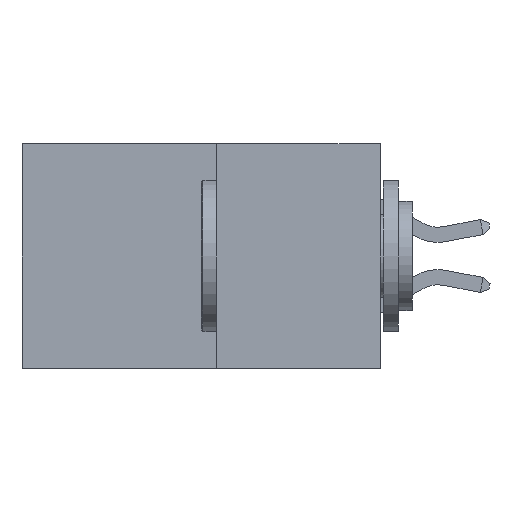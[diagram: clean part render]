
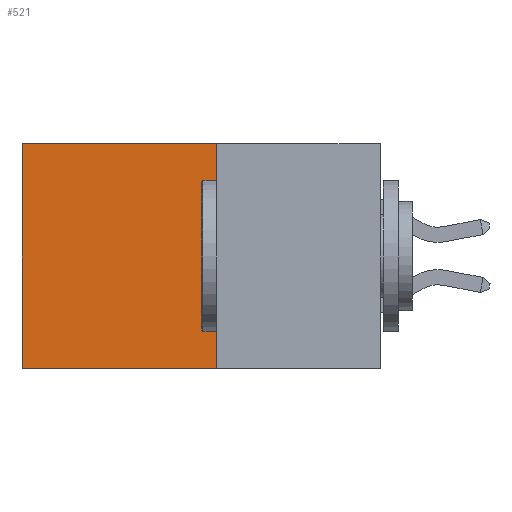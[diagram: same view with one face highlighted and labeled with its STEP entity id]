
A CAD part, left-side view. The second image highlights one B-rep face of the part: STEP entity #521.
In plain terms, the highlighted planar face has unit normal (-1, 0, 0).
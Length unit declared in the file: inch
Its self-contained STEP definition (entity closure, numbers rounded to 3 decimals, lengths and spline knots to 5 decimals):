
#521 = ADVANCED_FACE ( 'NONE', ( #11452 ), #2198, .F. ) ;
#563 = LINE ( 'NONE', #14332, #9038 ) ;
#1835 = VERTEX_POINT ( 'NONE', #4937 ) ;
#1877 = LINE ( 'NONE', #12986, #18671 ) ;
#2198 = PLANE ( 'NONE',  #16958 ) ;
#2316 = VECTOR ( 'NONE', #6111, 39.37008 ) ;
#2843 = LINE ( 'NONE', #6462, #2316 ) ;
#2913 = ORIENTED_EDGE ( 'NONE', *, *, #20749, .T. ) ;
#3268 = CARTESIAN_POINT ( 'NONE',  ( 0.277, 0.59, -0.37 ) ) ;
#3866 = ORIENTED_EDGE ( 'NONE', *, *, #10533, .T. ) ;
#4174 = EDGE_LOOP ( 'NONE', ( #3866, #16039, #15966, #2913 ) ) ;
#4552 = DIRECTION ( 'NONE',  ( 0., 1., 0. ) ) ;
#4937 = CARTESIAN_POINT ( 'NONE',  ( 0.277, 0.59, 0. ) ) ;
#6039 = DIRECTION ( 'NONE',  ( 1., 0., 0. ) ) ;
#6047 = CARTESIAN_POINT ( 'NONE',  ( 0.277, 0.27, -0.37 ) ) ;
#6111 = DIRECTION ( 'NONE',  ( 0., 0., -1. ) ) ;
#6462 = CARTESIAN_POINT ( 'NONE',  ( 0.277, 0.59, -0.37 ) ) ;
#7021 = CARTESIAN_POINT ( 'NONE',  ( 0.277, 0.27, -0.37 ) ) ;
#7268 = VECTOR ( 'NONE', #20323, 39.37008 ) ;
#9038 = VECTOR ( 'NONE', #11083, 39.37008 ) ;
#10260 = VERTEX_POINT ( 'NONE', #12584 ) ;
#10533 = EDGE_CURVE ( 'NONE', #1835, #16772, #2843, .T. ) ;
#10762 = CARTESIAN_POINT ( 'NONE',  ( 0.277, 0.27, 0. ) ) ;
#11035 = DIRECTION ( 'NONE',  ( 0., 0., -1. ) ) ;
#11083 = DIRECTION ( 'NONE',  ( 0., 1., 0. ) ) ;
#11452 = FACE_OUTER_BOUND ( 'NONE', #4174, .T. ) ;
#12584 = CARTESIAN_POINT ( 'NONE',  ( 0.277, 0.27, -0.37 ) ) ;
#12986 = CARTESIAN_POINT ( 'NONE',  ( 0.277, 0.27, 0. ) ) ;
#13469 = EDGE_CURVE ( 'NONE', #17388, #10260, #15726, .T. ) ;
#14332 = CARTESIAN_POINT ( 'NONE',  ( 0.277, 0.27, -0.37 ) ) ;
#15726 = LINE ( 'NONE', #7021, #7268 ) ;
#15820 = EDGE_CURVE ( 'NONE', #10260, #16772, #563, .T. ) ;
#15966 = ORIENTED_EDGE ( 'NONE', *, *, #13469, .F. ) ;
#16039 = ORIENTED_EDGE ( 'NONE', *, *, #15820, .F. ) ;
#16772 = VERTEX_POINT ( 'NONE', #3268 ) ;
#16958 = AXIS2_PLACEMENT_3D ( 'NONE', #6047, #6039, #11035 ) ;
#17388 = VERTEX_POINT ( 'NONE', #10762 ) ;
#18671 = VECTOR ( 'NONE', #4552, 39.37008 ) ;
#20323 = DIRECTION ( 'NONE',  ( 0., 0., -1. ) ) ;
#20749 = EDGE_CURVE ( 'NONE', #17388, #1835, #1877, .T. ) ;
